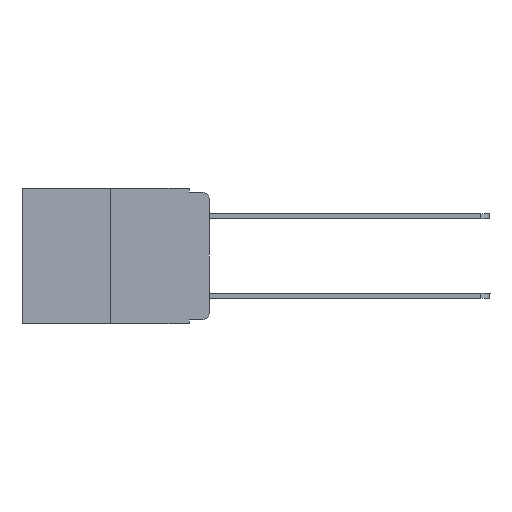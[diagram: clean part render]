
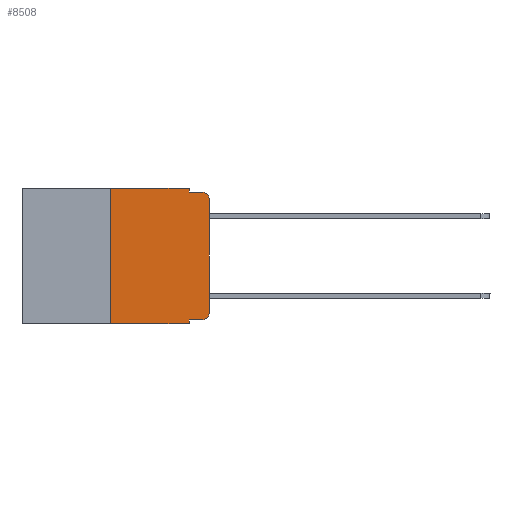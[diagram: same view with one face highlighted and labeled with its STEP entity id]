
A CAD part, left-side view. The second image highlights one B-rep face of the part: STEP entity #8508.
In plain terms, the highlighted planar face has unit normal (-1, 0, 0).
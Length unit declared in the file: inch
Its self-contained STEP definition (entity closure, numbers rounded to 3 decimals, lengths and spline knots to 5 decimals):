
#20 = VERTEX_POINT ( 'NONE', #3233 ) ;
#109 = VECTOR ( 'NONE', #669, 39.37008 ) ;
#209 = ORIENTED_EDGE ( 'NONE', *, *, #5286, .T. ) ;
#211 = ORIENTED_EDGE ( 'NONE', *, *, #7912, .F. ) ;
#403 = VERTEX_POINT ( 'NONE', #10476 ) ;
#483 = EDGE_CURVE ( 'NONE', #14042, #11512, #11032, .T. ) ;
#669 = DIRECTION ( 'NONE',  ( 0., 0., 1. ) ) ;
#1073 = AXIS2_PLACEMENT_3D ( 'NONE', #13218, #2248, #1352 ) ;
#1352 = DIRECTION ( 'NONE',  ( 0., 0., -1. ) ) ;
#1798 = ORIENTED_EDGE ( 'NONE', *, *, #11786, .F. ) ;
#2176 = FACE_OUTER_BOUND ( 'NONE', #3354, .T. ) ;
#2180 = CARTESIAN_POINT ( 'NONE',  ( 0., 0.02, -0.313 ) ) ;
#2248 = DIRECTION ( 'NONE',  ( -1., 0., 0. ) ) ;
#2417 = DIRECTION ( 'NONE',  ( 0., 0., -1. ) ) ;
#2773 = LINE ( 'NONE', #11325, #4661 ) ;
#3233 = CARTESIAN_POINT ( 'NONE',  ( 0., 0.25, 0. ) ) ;
#3354 = EDGE_LOOP ( 'NONE', ( #209, #7643, #211, #3845, #1798, #10223, #8816, #10002, #8364, #9975 ) ) ;
#3523 = LINE ( 'NONE', #4632, #3784 ) ;
#3784 = VECTOR ( 'NONE', #10891, 39.37008 ) ;
#3845 = ORIENTED_EDGE ( 'NONE', *, *, #5436, .F. ) ;
#3925 = CARTESIAN_POINT ( 'NONE',  ( 0., 0.25, -0.343 ) ) ;
#4183 = VERTEX_POINT ( 'NONE', #7366 ) ;
#4339 = DIRECTION ( 'NONE',  ( 0., -1., 0. ) ) ;
#4632 = CARTESIAN_POINT ( 'NONE',  ( 0., 0.25, 0. ) ) ;
#4651 = LINE ( 'NONE', #15677, #11900 ) ;
#4661 = VECTOR ( 'NONE', #14880, 39.37008 ) ;
#5055 = CARTESIAN_POINT ( 'NONE',  ( 0., 0., -0.03 ) ) ;
#5286 = EDGE_CURVE ( 'NONE', #4183, #14042, #7940, .T. ) ;
#5436 = EDGE_CURVE ( 'NONE', #14600, #403, #4651, .T. ) ;
#5450 = CARTESIAN_POINT ( 'NONE',  ( 0., 0.473, 0. ) ) ;
#6018 = CARTESIAN_POINT ( 'NONE',  ( 0., 0.051, -0.343 ) ) ;
#6233 = CIRCLE ( 'NONE', #7037, 0.02 ) ;
#7037 = AXIS2_PLACEMENT_3D ( 'NONE', #2180, #12991, #10568 ) ;
#7300 = VECTOR ( 'NONE', #9157, 39.37008 ) ;
#7366 = CARTESIAN_POINT ( 'NONE',  ( 0., 0., -0.313 ) ) ;
#7643 = ORIENTED_EDGE ( 'NONE', *, *, #483, .T. ) ;
#7868 = CARTESIAN_POINT ( 'NONE',  ( 0., 0.051, -0.01 ) ) ;
#7912 = EDGE_CURVE ( 'NONE', #403, #11512, #12758, .T. ) ;
#7940 = LINE ( 'NONE', #12843, #109 ) ;
#7973 = CARTESIAN_POINT ( 'NONE',  ( 0., 0.02, -0.01 ) ) ;
#7995 = DIRECTION ( 'NONE',  ( 1., 0., 0. ) ) ;
#8112 = CARTESIAN_POINT ( 'NONE',  ( 0., 0.473, -0.343 ) ) ;
#8199 = VERTEX_POINT ( 'NONE', #6018 ) ;
#8273 = VERTEX_POINT ( 'NONE', #9774 ) ;
#8327 = VERTEX_POINT ( 'NONE', #13704 ) ;
#8364 = ORIENTED_EDGE ( 'NONE', *, *, #12658, .T. ) ;
#8412 = LINE ( 'NONE', #15662, #15784 ) ;
#8430 = DIRECTION ( 'NONE',  ( 0., 0., -1. ) ) ;
#8508 = ADVANCED_FACE ( 'NONE', ( #2176 ), #15586, .F. ) ;
#8710 = EDGE_CURVE ( 'NONE', #9689, #20, #3523, .T. ) ;
#8719 = CARTESIAN_POINT ( 'NONE',  ( 0., 0.051, 0. ) ) ;
#8816 = ORIENTED_EDGE ( 'NONE', *, *, #13761, .T. ) ;
#9157 = DIRECTION ( 'NONE',  ( 0., -1., 0. ) ) ;
#9689 = VERTEX_POINT ( 'NONE', #3925 ) ;
#9698 = LINE ( 'NONE', #15846, #11322 ) ;
#9734 = EDGE_CURVE ( 'NONE', #8273, #4183, #6233, .T. ) ;
#9774 = CARTESIAN_POINT ( 'NONE',  ( 0., 0.02, -0.333 ) ) ;
#9826 = VECTOR ( 'NONE', #4339, 39.37008 ) ;
#9975 = ORIENTED_EDGE ( 'NONE', *, *, #9734, .T. ) ;
#10002 = ORIENTED_EDGE ( 'NONE', *, *, #14417, .F. ) ;
#10223 = ORIENTED_EDGE ( 'NONE', *, *, #8710, .F. ) ;
#10476 = CARTESIAN_POINT ( 'NONE',  ( 0., 0.051, -0.01 ) ) ;
#10568 = DIRECTION ( 'NONE',  ( 0., 0., -1. ) ) ;
#10586 = LINE ( 'NONE', #8112, #9826 ) ;
#10891 = DIRECTION ( 'NONE',  ( 0., 0., 1. ) ) ;
#11032 = CIRCLE ( 'NONE', #1073, 0.02 ) ;
#11322 = VECTOR ( 'NONE', #15766, 39.37008 ) ;
#11325 = CARTESIAN_POINT ( 'NONE',  ( 0., 0.473, 0. ) ) ;
#11512 = VERTEX_POINT ( 'NONE', #7973 ) ;
#11786 = EDGE_CURVE ( 'NONE', #20, #14600, #2773, .T. ) ;
#11900 = VECTOR ( 'NONE', #8430, 39.37008 ) ;
#12006 = AXIS2_PLACEMENT_3D ( 'NONE', #5450, #7995, #14105 ) ;
#12658 = EDGE_CURVE ( 'NONE', #8327, #8273, #9698, .T. ) ;
#12758 = LINE ( 'NONE', #7868, #7300 ) ;
#12843 = CARTESIAN_POINT ( 'NONE',  ( 0., 0., 0. ) ) ;
#12991 = DIRECTION ( 'NONE',  ( -1., 0., 0. ) ) ;
#13218 = CARTESIAN_POINT ( 'NONE',  ( 0., 0.02, -0.03 ) ) ;
#13704 = CARTESIAN_POINT ( 'NONE',  ( 0., 0.051, -0.333 ) ) ;
#13761 = EDGE_CURVE ( 'NONE', #9689, #8199, #10586, .T. ) ;
#14042 = VERTEX_POINT ( 'NONE', #5055 ) ;
#14105 = DIRECTION ( 'NONE',  ( 0., 0., -1. ) ) ;
#14417 = EDGE_CURVE ( 'NONE', #8327, #8199, #8412, .T. ) ;
#14600 = VERTEX_POINT ( 'NONE', #8719 ) ;
#14880 = DIRECTION ( 'NONE',  ( 0., -1., 0. ) ) ;
#15586 = PLANE ( 'NONE',  #12006 ) ;
#15662 = CARTESIAN_POINT ( 'NONE',  ( 0., 0.051, 0. ) ) ;
#15677 = CARTESIAN_POINT ( 'NONE',  ( 0., 0.051, 0. ) ) ;
#15766 = DIRECTION ( 'NONE',  ( 0., -1., 0. ) ) ;
#15784 = VECTOR ( 'NONE', #2417, 39.37008 ) ;
#15846 = CARTESIAN_POINT ( 'NONE',  ( 0., 0.051, -0.333 ) ) ;
